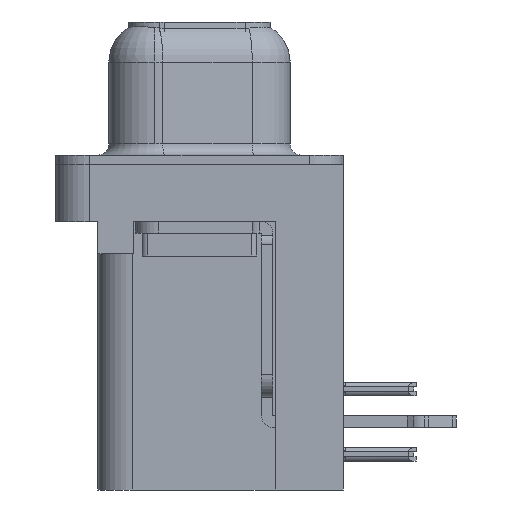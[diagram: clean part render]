
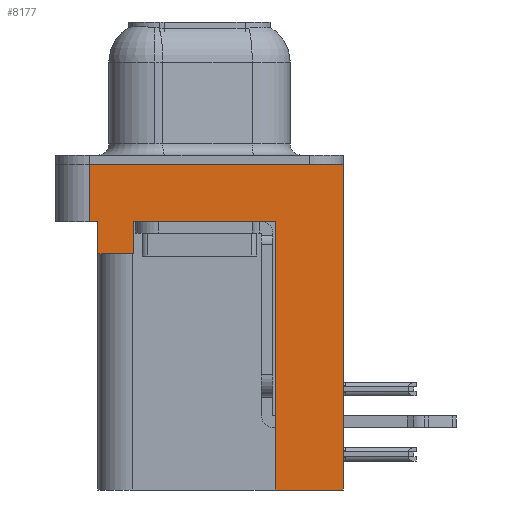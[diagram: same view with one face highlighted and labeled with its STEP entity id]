
A CAD part, left-side view. The second image highlights one B-rep face of the part: STEP entity #8177.
In plain terms, the highlighted planar face has unit normal (-1, 0, 0).
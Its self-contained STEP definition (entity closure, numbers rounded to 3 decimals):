
#100 = LINE ( 'NONE', #2474, #896 ) ;
#272 = VERTEX_POINT ( 'NONE', #21306 ) ;
#694 = DIRECTION ( 'NONE',  ( 0., -1., 0. ) ) ;
#812 = EDGE_CURVE ( 'NONE', #5305, #1735, #8285, .T. ) ;
#856 = DIRECTION ( 'NONE',  ( 0., 0., 1. ) ) ;
#896 = VECTOR ( 'NONE', #27390, 1000. ) ;
#1007 = VERTEX_POINT ( 'NONE', #17470 ) ;
#1735 = VERTEX_POINT ( 'NONE', #27794 ) ;
#1833 = VERTEX_POINT ( 'NONE', #10018 ) ;
#2474 = CARTESIAN_POINT ( 'NONE',  ( -3., 4.425, -3.9 ) ) ;
#2523 = EDGE_CURVE ( 'NONE', #5305, #27201, #100, .T. ) ;
#3084 = ORIENTED_EDGE ( 'NONE', *, *, #24868, .F. ) ;
#3227 = VERTEX_POINT ( 'NONE', #22116 ) ;
#3301 = EDGE_CURVE ( 'NONE', #272, #19571, #19739, .T. ) ;
#4281 = CARTESIAN_POINT ( 'NONE',  ( -3., -6.275, 0. ) ) ;
#4816 = CARTESIAN_POINT ( 'NONE',  ( -3., 2.895, -3.9 ) ) ;
#5305 = VERTEX_POINT ( 'NONE', #4816 ) ;
#5698 = ORIENTED_EDGE ( 'NONE', *, *, #15379, .T. ) ;
#6199 = CARTESIAN_POINT ( 'NONE',  ( -3., -6.275, -2.5 ) ) ;
#6492 = LINE ( 'NONE', #28765, #11252 ) ;
#6782 = CARTESIAN_POINT ( 'NONE',  ( -3., 4.425, -3.9 ) ) ;
#6857 = LINE ( 'NONE', #16216, #21991 ) ;
#8177 = ADVANCED_FACE ( 'NONE', ( #11876 ), #20650, .T. ) ;
#8285 = LINE ( 'NONE', #19410, #10742 ) ;
#8326 = LINE ( 'NONE', #24208, #14628 ) ;
#8472 = DIRECTION ( 'NONE',  ( 0., 0., 1. ) ) ;
#9406 = VECTOR ( 'NONE', #14880, 1000. ) ;
#9707 = DIRECTION ( 'NONE',  ( 0., 0., 1. ) ) ;
#9742 = CARTESIAN_POINT ( 'NONE',  ( -3., -3.295, -14.2 ) ) ;
#9867 = ORIENTED_EDGE ( 'NONE', *, *, #812, .T. ) ;
#9941 = EDGE_CURVE ( 'NONE', #1735, #1007, #6492, .T. ) ;
#9988 = VECTOR ( 'NONE', #9707, 1000. ) ;
#10018 = CARTESIAN_POINT ( 'NONE',  ( -3., -3.295, -14.2 ) ) ;
#10672 = EDGE_LOOP ( 'NONE', ( #15722, #12346, #5698, #16263, #27354, #9867, #27007, #10748, #3084, #25649 ) ) ;
#10742 = VECTOR ( 'NONE', #856, 1000. ) ;
#10748 = ORIENTED_EDGE ( 'NONE', *, *, #13728, .F. ) ;
#10957 = DIRECTION ( 'NONE',  ( 0., 0., 1. ) ) ;
#11224 = CARTESIAN_POINT ( 'NONE',  ( -3., 4.775, -2.5 ) ) ;
#11252 = VECTOR ( 'NONE', #21961, 1000. ) ;
#11689 = LINE ( 'NONE', #25629, #27478 ) ;
#11876 = FACE_OUTER_BOUND ( 'NONE', #10672, .T. ) ;
#12016 = DIRECTION ( 'NONE',  ( 0., 0., 1. ) ) ;
#12346 = ORIENTED_EDGE ( 'NONE', *, *, #16202, .F. ) ;
#12500 = AXIS2_PLACEMENT_3D ( 'NONE', #25671, #16055, #12016 ) ;
#12828 = CARTESIAN_POINT ( 'NONE',  ( -3., 4.425, -2.5 ) ) ;
#13728 = EDGE_CURVE ( 'NONE', #1833, #1007, #8326, .T. ) ;
#14628 = VECTOR ( 'NONE', #8472, 1000. ) ;
#14880 = DIRECTION ( 'NONE',  ( 0., 1., 0. ) ) ;
#15379 = EDGE_CURVE ( 'NONE', #24560, #26222, #11689, .T. ) ;
#15722 = ORIENTED_EDGE ( 'NONE', *, *, #3301, .F. ) ;
#15922 = DIRECTION ( 'NONE',  ( 0., 0., 1. ) ) ;
#16055 = DIRECTION ( 'NONE',  ( -1., 0., 0. ) ) ;
#16202 = EDGE_CURVE ( 'NONE', #24560, #272, #20097, .T. ) ;
#16216 = CARTESIAN_POINT ( 'NONE',  ( -3., 4.425, -3.9 ) ) ;
#16263 = ORIENTED_EDGE ( 'NONE', *, *, #21547, .F. ) ;
#17470 = CARTESIAN_POINT ( 'NONE',  ( -3., -3.295, -2.5 ) ) ;
#18404 = EDGE_CURVE ( 'NONE', #3227, #19571, #28757, .T. ) ;
#19075 = VECTOR ( 'NONE', #10957, 1000. ) ;
#19410 = CARTESIAN_POINT ( 'NONE',  ( -3., 2.895, -3.9 ) ) ;
#19571 = VERTEX_POINT ( 'NONE', #4281 ) ;
#19739 = LINE ( 'NONE', #24482, #21380 ) ;
#19764 = LINE ( 'NONE', #9742, #9406 ) ;
#20097 = LINE ( 'NONE', #27775, #9988 ) ;
#20650 = PLANE ( 'NONE',  #12500 ) ;
#21306 = CARTESIAN_POINT ( 'NONE',  ( -3., 4.775, 0. ) ) ;
#21380 = VECTOR ( 'NONE', #24925, 1000. ) ;
#21547 = EDGE_CURVE ( 'NONE', #27201, #26222, #6857, .T. ) ;
#21961 = DIRECTION ( 'NONE',  ( 0., -1., 0. ) ) ;
#21991 = VECTOR ( 'NONE', #15922, 1000. ) ;
#22116 = CARTESIAN_POINT ( 'NONE',  ( -3., -6.275, -14.2 ) ) ;
#24208 = CARTESIAN_POINT ( 'NONE',  ( -3., -3.295, -14.2 ) ) ;
#24482 = CARTESIAN_POINT ( 'NONE',  ( -3., -6.275, 0. ) ) ;
#24560 = VERTEX_POINT ( 'NONE', #11224 ) ;
#24868 = EDGE_CURVE ( 'NONE', #3227, #1833, #19764, .T. ) ;
#24925 = DIRECTION ( 'NONE',  ( 0., -1., 0. ) ) ;
#25629 = CARTESIAN_POINT ( 'NONE',  ( -3., -6.275, -2.5 ) ) ;
#25649 = ORIENTED_EDGE ( 'NONE', *, *, #18404, .T. ) ;
#25671 = CARTESIAN_POINT ( 'NONE',  ( -3., -6.275, -2.5 ) ) ;
#26222 = VERTEX_POINT ( 'NONE', #12828 ) ;
#27007 = ORIENTED_EDGE ( 'NONE', *, *, #9941, .T. ) ;
#27201 = VERTEX_POINT ( 'NONE', #6782 ) ;
#27354 = ORIENTED_EDGE ( 'NONE', *, *, #2523, .F. ) ;
#27390 = DIRECTION ( 'NONE',  ( 0., 1., 0. ) ) ;
#27478 = VECTOR ( 'NONE', #694, 1000. ) ;
#27775 = CARTESIAN_POINT ( 'NONE',  ( -3., 4.775, -2.5 ) ) ;
#27794 = CARTESIAN_POINT ( 'NONE',  ( -3., 2.895, -2.5 ) ) ;
#28757 = LINE ( 'NONE', #6199, #19075 ) ;
#28765 = CARTESIAN_POINT ( 'NONE',  ( -3., -6.275, -2.5 ) ) ;
